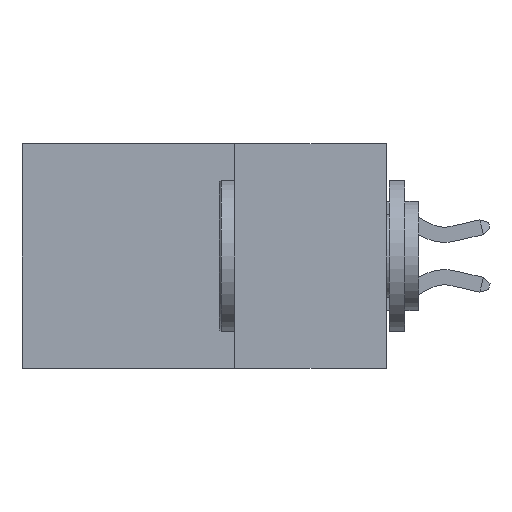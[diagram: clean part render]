
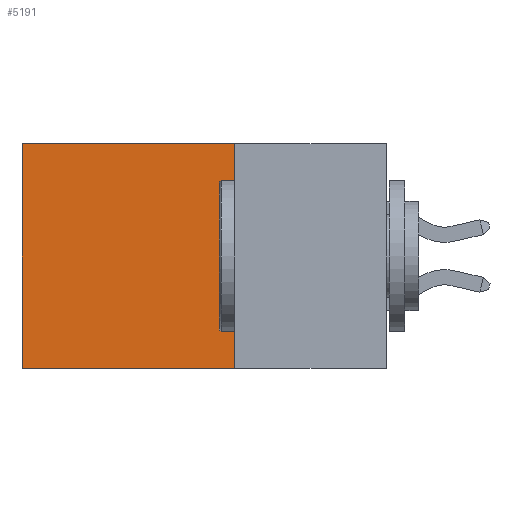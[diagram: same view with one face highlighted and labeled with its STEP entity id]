
A CAD part, left-side view. The second image highlights one B-rep face of the part: STEP entity #5191.
In plain terms, the highlighted planar face has unit normal (-1, 0, 0).
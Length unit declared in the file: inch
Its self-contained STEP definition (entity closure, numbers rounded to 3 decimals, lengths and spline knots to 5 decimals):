
#118 = EDGE_CURVE ( 'NONE', #6951, #5537, #7427, .T. ) ;
#144 = CARTESIAN_POINT ( 'NONE',  ( 0.2615, 0.25, 0. ) ) ;
#279 = EDGE_CURVE ( 'NONE', #6903, #8780, #6326, .T. ) ;
#281 = CARTESIAN_POINT ( 'NONE',  ( 0.2615, 0.6, 0. ) ) ;
#798 = FACE_OUTER_BOUND ( 'NONE', #9985, .T. ) ;
#1668 = CARTESIAN_POINT ( 'NONE',  ( 0.2615, 0.25, -0.37 ) ) ;
#1872 = DIRECTION ( 'NONE',  ( 0., 1., 0. ) ) ;
#2533 = ORIENTED_EDGE ( 'NONE', *, *, #118, .F. ) ;
#2646 = CARTESIAN_POINT ( 'NONE',  ( 0.2615, 0.6, -0.37 ) ) ;
#3050 = VECTOR ( 'NONE', #10097, 39.37008 ) ;
#3650 = VECTOR ( 'NONE', #9304, 39.37008 ) ;
#4110 = EDGE_CURVE ( 'NONE', #5537, #8780, #6935, .T. ) ;
#4666 = CARTESIAN_POINT ( 'NONE',  ( 0.2615, 0.6, -0.37 ) ) ;
#4681 = ORIENTED_EDGE ( 'NONE', *, *, #279, .T. ) ;
#4977 = ORIENTED_EDGE ( 'NONE', *, *, #10489, .T. ) ;
#5155 = DIRECTION ( 'NONE',  ( 0., 0., -1. ) ) ;
#5191 = ADVANCED_FACE ( 'NONE', ( #798 ), #9376, .F. ) ;
#5249 = CARTESIAN_POINT ( 'NONE',  ( 0.2615, 0.25, -0.37 ) ) ;
#5537 = VERTEX_POINT ( 'NONE', #7199 ) ;
#6326 = LINE ( 'NONE', #2646, #3650 ) ;
#6903 = VERTEX_POINT ( 'NONE', #281 ) ;
#6935 = LINE ( 'NONE', #1668, #9011 ) ;
#6951 = VERTEX_POINT ( 'NONE', #144 ) ;
#7044 = ORIENTED_EDGE ( 'NONE', *, *, #4110, .F. ) ;
#7199 = CARTESIAN_POINT ( 'NONE',  ( 0.2615, 0.25, -0.37 ) ) ;
#7427 = LINE ( 'NONE', #5249, #11426 ) ;
#8358 = CARTESIAN_POINT ( 'NONE',  ( 0.2615, 0.25, 0. ) ) ;
#8780 = VERTEX_POINT ( 'NONE', #4666 ) ;
#9011 = VECTOR ( 'NONE', #1872, 39.37008 ) ;
#9299 = DIRECTION ( 'NONE',  ( 0., 0., -1. ) ) ;
#9304 = DIRECTION ( 'NONE',  ( 0., 0., -1. ) ) ;
#9309 = DIRECTION ( 'NONE',  ( 1., 0., 0. ) ) ;
#9336 = CARTESIAN_POINT ( 'NONE',  ( 0.2615, 0.25, -0.37 ) ) ;
#9376 = PLANE ( 'NONE',  #11079 ) ;
#9985 = EDGE_LOOP ( 'NONE', ( #4681, #7044, #2533, #4977 ) ) ;
#10097 = DIRECTION ( 'NONE',  ( 0., 1., 0. ) ) ;
#10121 = LINE ( 'NONE', #8358, #3050 ) ;
#10489 = EDGE_CURVE ( 'NONE', #6951, #6903, #10121, .T. ) ;
#11079 = AXIS2_PLACEMENT_3D ( 'NONE', #9336, #9309, #9299 ) ;
#11426 = VECTOR ( 'NONE', #5155, 39.37008 ) ;
